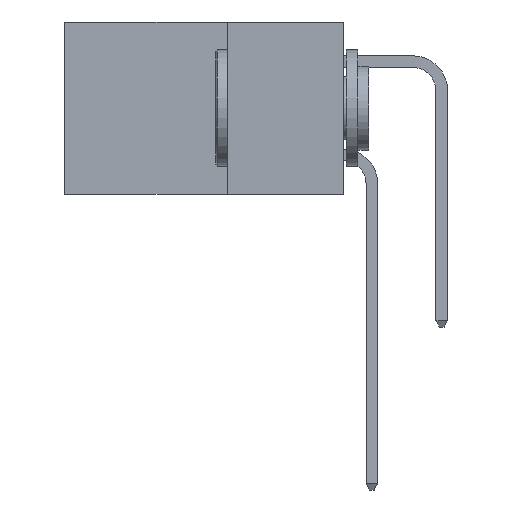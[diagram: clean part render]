
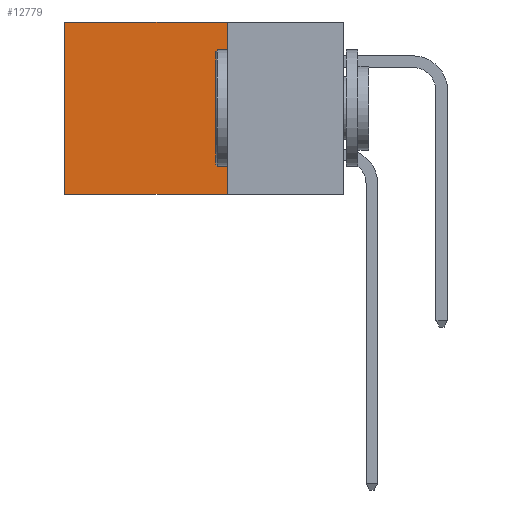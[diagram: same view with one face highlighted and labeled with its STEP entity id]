
A CAD part, left-side view. The second image highlights one B-rep face of the part: STEP entity #12779.
In plain terms, the highlighted planar face has unit normal (-1, 0, 0).
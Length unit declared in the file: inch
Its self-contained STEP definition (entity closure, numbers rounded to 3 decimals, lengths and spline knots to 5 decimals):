
#382 = EDGE_CURVE ( 'NONE', #17992, #3397, #10790, .T. ) ;
#2508 = ORIENTED_EDGE ( 'NONE', *, *, #15940, .F. ) ;
#2602 = DIRECTION ( 'NONE',  ( 0., 0., -1. ) ) ;
#2829 = CARTESIAN_POINT ( 'NONE',  ( 0.2615, 0.6, 0. ) ) ;
#3273 = LINE ( 'NONE', #3535, #20972 ) ;
#3397 = VERTEX_POINT ( 'NONE', #19860 ) ;
#3490 = FACE_OUTER_BOUND ( 'NONE', #12165, .T. ) ;
#3535 = CARTESIAN_POINT ( 'NONE',  ( 0.2615, 0.25, 0. ) ) ;
#3662 = DIRECTION ( 'NONE',  ( 0., 1., 0. ) ) ;
#5104 = PLANE ( 'NONE',  #11585 ) ;
#5135 = EDGE_CURVE ( 'NONE', #14024, #3397, #18313, .T. ) ;
#6115 = VERTEX_POINT ( 'NONE', #14677 ) ;
#6193 = VECTOR ( 'NONE', #2602, 39.37008 ) ;
#6639 = ORIENTED_EDGE ( 'NONE', *, *, #5135, .F. ) ;
#6844 = DIRECTION ( 'NONE',  ( 1., 0., 0. ) ) ;
#8550 = CARTESIAN_POINT ( 'NONE',  ( 0.2615, 0.6, -0.37 ) ) ;
#10790 = LINE ( 'NONE', #8550, #6193 ) ;
#11585 = AXIS2_PLACEMENT_3D ( 'NONE', #17125, #6844, #18801 ) ;
#12165 = EDGE_LOOP ( 'NONE', ( #14396, #6639, #2508, #17872 ) ) ;
#12291 = LINE ( 'NONE', #14622, #20765 ) ;
#12779 = ADVANCED_FACE ( 'NONE', ( #3490 ), #5104, .F. ) ;
#13452 = CARTESIAN_POINT ( 'NONE',  ( 0.2615, 0.25, -0.37 ) ) ;
#13925 = DIRECTION ( 'NONE',  ( 0., 1., 0. ) ) ;
#14024 = VERTEX_POINT ( 'NONE', #13452 ) ;
#14039 = CARTESIAN_POINT ( 'NONE',  ( 0.2615, 0.25, -0.37 ) ) ;
#14364 = VECTOR ( 'NONE', #3662, 39.37008 ) ;
#14396 = ORIENTED_EDGE ( 'NONE', *, *, #382, .T. ) ;
#14622 = CARTESIAN_POINT ( 'NONE',  ( 0.2615, 0.25, -0.37 ) ) ;
#14677 = CARTESIAN_POINT ( 'NONE',  ( 0.2615, 0.25, 0. ) ) ;
#15940 = EDGE_CURVE ( 'NONE', #6115, #14024, #12291, .T. ) ;
#16319 = DIRECTION ( 'NONE',  ( 0., 0., -1. ) ) ;
#16928 = EDGE_CURVE ( 'NONE', #6115, #17992, #3273, .T. ) ;
#17125 = CARTESIAN_POINT ( 'NONE',  ( 0.2615, 0.25, -0.37 ) ) ;
#17872 = ORIENTED_EDGE ( 'NONE', *, *, #16928, .T. ) ;
#17992 = VERTEX_POINT ( 'NONE', #2829 ) ;
#18313 = LINE ( 'NONE', #14039, #14364 ) ;
#18801 = DIRECTION ( 'NONE',  ( 0., 0., -1. ) ) ;
#19860 = CARTESIAN_POINT ( 'NONE',  ( 0.2615, 0.6, -0.37 ) ) ;
#20765 = VECTOR ( 'NONE', #16319, 39.37008 ) ;
#20972 = VECTOR ( 'NONE', #13925, 39.37008 ) ;
